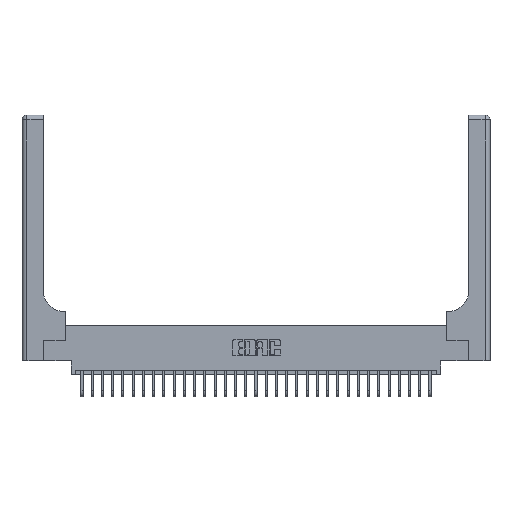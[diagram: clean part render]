
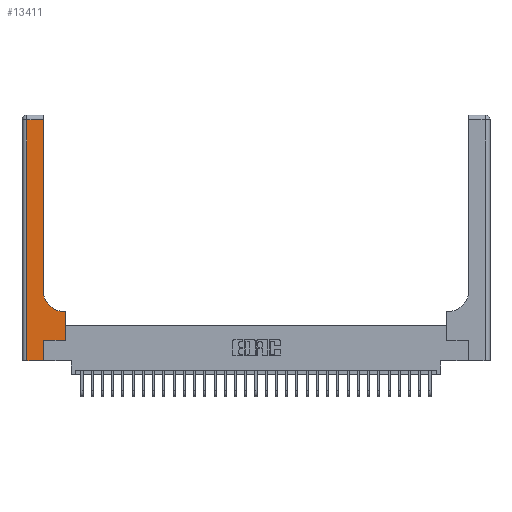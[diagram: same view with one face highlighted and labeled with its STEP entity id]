
A CAD part, top view. The second image highlights one B-rep face of the part: STEP entity #13411.
In plain terms, the highlighted planar face has unit normal (0, 0, 1).
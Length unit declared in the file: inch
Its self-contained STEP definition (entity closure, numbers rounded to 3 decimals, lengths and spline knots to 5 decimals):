
#109 = ORIENTED_EDGE ( 'NONE', *, *, #7760, .T. ) ;
#569 = CARTESIAN_POINT ( 'NONE',  ( 0.528, 0.25, 0.37 ) ) ;
#678 = CARTESIAN_POINT ( 'NONE',  ( 0.265, 0., 0.37 ) ) ;
#849 = ORIENTED_EDGE ( 'NONE', *, *, #2505, .T. ) ;
#1279 = LINE ( 'NONE', #2322, #12215 ) ;
#1500 = LINE ( 'NONE', #22879, #23840 ) ;
#2061 = VERTEX_POINT ( 'NONE', #20242 ) ;
#2247 = EDGE_LOOP ( 'NONE', ( #849, #2727, #10377, #26903, #2899, #9279, #109, #7415, #17864 ) ) ;
#2322 = CARTESIAN_POINT ( 'NONE',  ( 0.06, 3., 0.37 ) ) ;
#2505 = EDGE_CURVE ( 'NONE', #17570, #5672, #12858, .T. ) ;
#2727 = ORIENTED_EDGE ( 'NONE', *, *, #16634, .T. ) ;
#2872 = VERTEX_POINT ( 'NONE', #13338 ) ;
#2899 = ORIENTED_EDGE ( 'NONE', *, *, #9181, .T. ) ;
#3519 = VECTOR ( 'NONE', #12481, 39.37008 ) ;
#4705 = CARTESIAN_POINT ( 'NONE',  ( 0.26, 3., 0.37 ) ) ;
#5544 = LINE ( 'NONE', #14673, #27858 ) ;
#5672 = VERTEX_POINT ( 'NONE', #10050 ) ;
#5730 = VECTOR ( 'NONE', #11676, 39.37008 ) ;
#6426 = LINE ( 'NONE', #678, #5730 ) ;
#6489 = DIRECTION ( 'NONE',  ( 0., 0., -1. ) ) ;
#7324 = PLANE ( 'NONE',  #25618 ) ;
#7415 = ORIENTED_EDGE ( 'NONE', *, *, #14982, .T. ) ;
#7760 = EDGE_CURVE ( 'NONE', #17305, #25224, #12999, .T. ) ;
#8027 = EDGE_CURVE ( 'NONE', #21210, #17570, #27098, .T. ) ;
#9143 = AXIS2_PLACEMENT_3D ( 'NONE', #19420, #6489, #21564 ) ;
#9181 = EDGE_CURVE ( 'NONE', #2872, #10115, #6426, .T. ) ;
#9279 = ORIENTED_EDGE ( 'NONE', *, *, #20445, .T. ) ;
#9327 = CARTESIAN_POINT ( 'NONE',  ( 0.06, 0., 0.37 ) ) ;
#9485 = DIRECTION ( 'NONE',  ( 0., 1., 0. ) ) ;
#9881 = CARTESIAN_POINT ( 'NONE',  ( 0.528, 0.6, 0.37 ) ) ;
#10050 = CARTESIAN_POINT ( 'NONE',  ( 0.26, 2.94, 0.37 ) ) ;
#10115 = VERTEX_POINT ( 'NONE', #26003 ) ;
#10234 = CARTESIAN_POINT ( 'NONE',  ( 0.26, 0.85, 0.37 ) ) ;
#10377 = ORIENTED_EDGE ( 'NONE', *, *, #24369, .T. ) ;
#11676 = DIRECTION ( 'NONE',  ( 0., 1., 0. ) ) ;
#11705 = CARTESIAN_POINT ( 'NONE',  ( 0., 3., 0.37 ) ) ;
#12215 = VECTOR ( 'NONE', #13344, 39.37008 ) ;
#12481 = DIRECTION ( 'NONE',  ( 1., 0., 0. ) ) ;
#12638 = LINE ( 'NONE', #18781, #16984 ) ;
#12858 = LINE ( 'NONE', #4705, #13548 ) ;
#12999 = LINE ( 'NONE', #15909, #23024 ) ;
#13338 = CARTESIAN_POINT ( 'NONE',  ( 0.265, 0., 0.37 ) ) ;
#13344 = DIRECTION ( 'NONE',  ( 0., -1., 0. ) ) ;
#13411 = ADVANCED_FACE ( 'NONE', ( #17139 ), #7324, .F. ) ;
#13525 = EDGE_CURVE ( 'NONE', #26358, #2872, #25168, .T. ) ;
#13548 = VECTOR ( 'NONE', #19840, 39.37008 ) ;
#14303 = DIRECTION ( 'NONE',  ( -1., 0., 0. ) ) ;
#14673 = CARTESIAN_POINT ( 'NONE',  ( 0.26, 0.6, 0.37 ) ) ;
#14982 = EDGE_CURVE ( 'NONE', #25224, #21210, #5544, .T. ) ;
#15909 = CARTESIAN_POINT ( 'NONE',  ( 0.528, 0.25, 0.37 ) ) ;
#16531 = DIRECTION ( 'NONE',  ( 1., 0., 0. ) ) ;
#16634 = EDGE_CURVE ( 'NONE', #5672, #2061, #12638, .T. ) ;
#16984 = VECTOR ( 'NONE', #20893, 39.37008 ) ;
#17139 = FACE_OUTER_BOUND ( 'NONE', #2247, .T. ) ;
#17305 = VERTEX_POINT ( 'NONE', #569 ) ;
#17570 = VERTEX_POINT ( 'NONE', #10234 ) ;
#17864 = ORIENTED_EDGE ( 'NONE', *, *, #8027, .T. ) ;
#18781 = CARTESIAN_POINT ( 'NONE',  ( 0., 2.94, 0.37 ) ) ;
#18958 = DIRECTION ( 'NONE',  ( -1., 0., 0. ) ) ;
#19184 = CARTESIAN_POINT ( 'NONE',  ( 0.51, 0.6, 0.37 ) ) ;
#19420 = CARTESIAN_POINT ( 'NONE',  ( 0.51, 0.85, 0.37 ) ) ;
#19840 = DIRECTION ( 'NONE',  ( 0., 1., 0. ) ) ;
#20242 = CARTESIAN_POINT ( 'NONE',  ( 0.06, 2.94, 0.37 ) ) ;
#20445 = EDGE_CURVE ( 'NONE', #10115, #17305, #1500, .T. ) ;
#20893 = DIRECTION ( 'NONE',  ( -1., 0., 0. ) ) ;
#21210 = VERTEX_POINT ( 'NONE', #19184 ) ;
#21564 = DIRECTION ( 'NONE',  ( 1., 0., 0. ) ) ;
#22879 = CARTESIAN_POINT ( 'NONE',  ( 0.265, 0.25, 0.37 ) ) ;
#23024 = VECTOR ( 'NONE', #9485, 39.37008 ) ;
#23840 = VECTOR ( 'NONE', #16531, 39.37008 ) ;
#24369 = EDGE_CURVE ( 'NONE', #2061, #26358, #1279, .T. ) ;
#25168 = LINE ( 'NONE', #25305, #3519 ) ;
#25224 = VERTEX_POINT ( 'NONE', #9881 ) ;
#25305 = CARTESIAN_POINT ( 'NONE',  ( 0., 0., 0.37 ) ) ;
#25618 = AXIS2_PLACEMENT_3D ( 'NONE', #11705, #26752, #14303 ) ;
#26003 = CARTESIAN_POINT ( 'NONE',  ( 0.265, 0.25, 0.37 ) ) ;
#26358 = VERTEX_POINT ( 'NONE', #9327 ) ;
#26752 = DIRECTION ( 'NONE',  ( 0., 0., -1. ) ) ;
#26903 = ORIENTED_EDGE ( 'NONE', *, *, #13525, .T. ) ;
#27098 = CIRCLE ( 'NONE', #9143, 0.25 ) ;
#27858 = VECTOR ( 'NONE', #18958, 39.37008 ) ;
